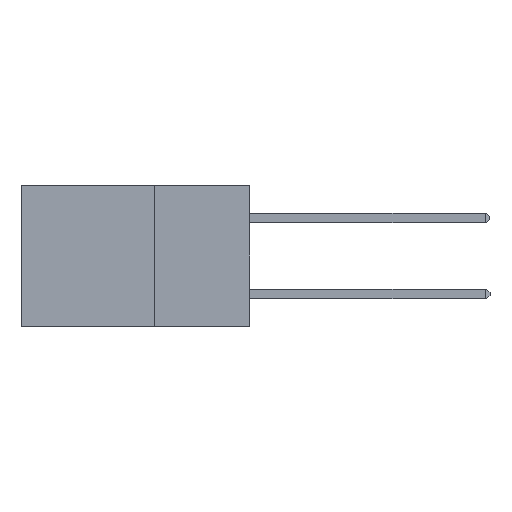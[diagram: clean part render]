
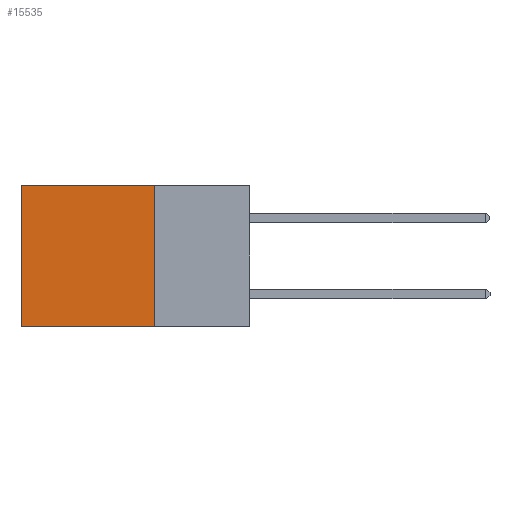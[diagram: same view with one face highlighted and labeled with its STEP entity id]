
A CAD part, left-side view. The second image highlights one B-rep face of the part: STEP entity #15535.
In plain terms, the highlighted planar face has unit normal (-1, 0, 0).
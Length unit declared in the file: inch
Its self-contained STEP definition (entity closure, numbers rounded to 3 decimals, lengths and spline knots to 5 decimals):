
#154 = ORIENTED_EDGE ( 'NONE', *, *, #8121, .F. ) ;
#877 = LINE ( 'NONE', #5919, #4759 ) ;
#1160 = PLANE ( 'NONE',  #3429 ) ;
#1491 = VERTEX_POINT ( 'NONE', #10768 ) ;
#2236 = VERTEX_POINT ( 'NONE', #17925 ) ;
#2684 = CARTESIAN_POINT ( 'NONE',  ( 0.2875, 0.6, 0. ) ) ;
#3429 = AXIS2_PLACEMENT_3D ( 'NONE', #6149, #18145, #7880 ) ;
#3629 = ORIENTED_EDGE ( 'NONE', *, *, #5604, .F. ) ;
#4205 = CARTESIAN_POINT ( 'NONE',  ( 0.2875, 0.25, -0.37 ) ) ;
#4283 = DIRECTION ( 'NONE',  ( 0., 1., 0. ) ) ;
#4327 = DIRECTION ( 'NONE',  ( 0., 0., -1. ) ) ;
#4759 = VECTOR ( 'NONE', #16239, 39.37008 ) ;
#5604 = EDGE_CURVE ( 'NONE', #7361, #2236, #20497, .T. ) ;
#5716 = LINE ( 'NONE', #12294, #10309 ) ;
#5919 = CARTESIAN_POINT ( 'NONE',  ( 0.2875, 0.25, 0. ) ) ;
#6149 = CARTESIAN_POINT ( 'NONE',  ( 0.2875, 0.25, 0. ) ) ;
#7361 = VERTEX_POINT ( 'NONE', #15003 ) ;
#7880 = DIRECTION ( 'NONE',  ( 0., 0., -1. ) ) ;
#7984 = VECTOR ( 'NONE', #4283, 39.37008 ) ;
#8121 = EDGE_CURVE ( 'NONE', #18650, #7361, #5716, .T. ) ;
#8779 = DIRECTION ( 'NONE',  ( 0., 0., -1. ) ) ;
#9130 = CARTESIAN_POINT ( 'NONE',  ( 0.2875, 0.25, 0. ) ) ;
#10309 = VECTOR ( 'NONE', #8779, 39.37008 ) ;
#10662 = EDGE_LOOP ( 'NONE', ( #13516, #3629, #154, #16625 ) ) ;
#10768 = CARTESIAN_POINT ( 'NONE',  ( 0.2875, 0.6, 0. ) ) ;
#12294 = CARTESIAN_POINT ( 'NONE',  ( 0.2875, 0.25, 0. ) ) ;
#12684 = LINE ( 'NONE', #2684, #20989 ) ;
#13516 = ORIENTED_EDGE ( 'NONE', *, *, #20986, .T. ) ;
#15003 = CARTESIAN_POINT ( 'NONE',  ( 0.2875, 0.25, -0.37 ) ) ;
#15535 = ADVANCED_FACE ( 'NONE', ( #21709 ), #1160, .F. ) ;
#15984 = EDGE_CURVE ( 'NONE', #18650, #1491, #877, .T. ) ;
#16239 = DIRECTION ( 'NONE',  ( 0., 1., 0. ) ) ;
#16625 = ORIENTED_EDGE ( 'NONE', *, *, #15984, .T. ) ;
#17925 = CARTESIAN_POINT ( 'NONE',  ( 0.2875, 0.6, -0.37 ) ) ;
#18145 = DIRECTION ( 'NONE',  ( 1., 0., 0. ) ) ;
#18650 = VERTEX_POINT ( 'NONE', #9130 ) ;
#20497 = LINE ( 'NONE', #4205, #7984 ) ;
#20986 = EDGE_CURVE ( 'NONE', #1491, #2236, #12684, .T. ) ;
#20989 = VECTOR ( 'NONE', #4327, 39.37008 ) ;
#21709 = FACE_OUTER_BOUND ( 'NONE', #10662, .T. ) ;
